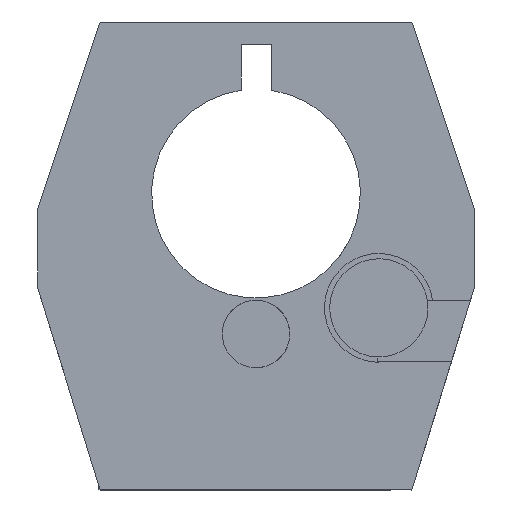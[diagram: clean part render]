
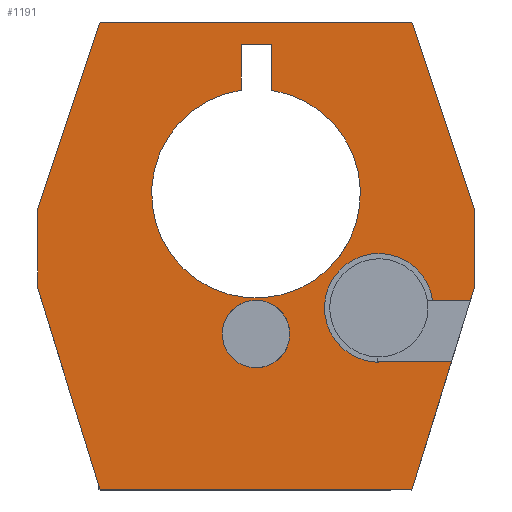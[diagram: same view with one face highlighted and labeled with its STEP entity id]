
A CAD part, front view. The second image highlights one B-rep face of the part: STEP entity #1191.
In plain terms, the highlighted planar face has unit normal (0, -1, 0).
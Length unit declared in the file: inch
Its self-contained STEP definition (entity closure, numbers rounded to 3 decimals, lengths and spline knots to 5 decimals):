
#20=FACE_BOUND('',#128,.T.);
#21=FACE_BOUND('',#129,.T.);
#63=FACE_OUTER_BOUND('',#127,.T.);
#127=EDGE_LOOP('',(#891,#892,#893,#894,#895,#896,#897,#898,#899,#900,#901,
#902,#903,#904,#905,#906));
#128=EDGE_LOOP('',(#907,#908,#909,#910));
#129=EDGE_LOOP('',(#911,#912));
#177=CIRCLE('',#1270,0.10827);
#178=CIRCLE('',#1271,0.10827);
#180=CIRCLE('',#1280,0.17421);
#181=CIRCLE('',#1282,0.33465);
#190=LINE('',#1648,#342);
#239=LINE('',#1763,#391);
#243=LINE('',#1770,#395);
#248=LINE('',#1830,#400);
#250=LINE('',#1836,#402);
#251=LINE('',#1838,#403);
#252=LINE('',#1840,#404);
#253=LINE('',#1842,#405);
#254=LINE('',#1844,#406);
#255=LINE('',#1846,#407);
#256=LINE('',#1848,#408);
#257=LINE('',#1850,#409);
#258=LINE('',#1851,#410);
#259=LINE('',#1853,#411);
#260=LINE('',#1854,#412);
#261=LINE('',#1859,#413);
#262=LINE('',#1861,#414);
#263=LINE('',#1862,#415);
#342=VECTOR('',#1333,0.3937);
#391=VECTOR('',#1432,0.3937);
#395=VECTOR('',#1438,0.3937);
#400=VECTOR('',#1463,0.3937);
#402=VECTOR('',#1471,0.3937);
#403=VECTOR('',#1472,0.3937);
#404=VECTOR('',#1473,0.3937);
#405=VECTOR('',#1474,0.3937);
#406=VECTOR('',#1475,0.3937);
#407=VECTOR('',#1476,0.3937);
#408=VECTOR('',#1477,0.3937);
#409=VECTOR('',#1478,0.3937);
#410=VECTOR('',#1479,0.3937);
#411=VECTOR('',#1480,0.3937);
#412=VECTOR('',#1481,0.3937);
#413=VECTOR('',#1484,0.3937);
#414=VECTOR('',#1485,0.3937);
#415=VECTOR('',#1486,0.3937);
#494=VERTEX_POINT('',#1645);
#495=VERTEX_POINT('',#1647);
#535=VERTEX_POINT('',#1760);
#536=VERTEX_POINT('',#1762);
#538=VERTEX_POINT('',#1768);
#539=VERTEX_POINT('',#1772);
#540=VERTEX_POINT('',#1773);
#546=VERTEX_POINT('',#1827);
#547=VERTEX_POINT('',#1829);
#548=VERTEX_POINT('',#1835);
#549=VERTEX_POINT('',#1837);
#550=VERTEX_POINT('',#1839);
#551=VERTEX_POINT('',#1841);
#552=VERTEX_POINT('',#1843);
#553=VERTEX_POINT('',#1845);
#554=VERTEX_POINT('',#1847);
#555=VERTEX_POINT('',#1849);
#556=VERTEX_POINT('',#1852);
#557=VERTEX_POINT('',#1855);
#558=VERTEX_POINT('',#1856);
#559=VERTEX_POINT('',#1858);
#560=VERTEX_POINT('',#1860);
#608=EDGE_CURVE('',#495,#494,#190,.T.);
#663=EDGE_CURVE('',#535,#536,#239,.T.);
#667=EDGE_CURVE('',#538,#535,#243,.T.);
#668=EDGE_CURVE('',#539,#540,#177,.T.);
#669=EDGE_CURVE('',#540,#539,#178,.T.);
#679=EDGE_CURVE('',#547,#546,#248,.T.);
#681=EDGE_CURVE('',#494,#547,#180,.T.);
#682=EDGE_CURVE('',#546,#548,#250,.T.);
#683=EDGE_CURVE('',#548,#549,#251,.T.);
#684=EDGE_CURVE('',#549,#550,#252,.T.);
#685=EDGE_CURVE('',#550,#551,#253,.T.);
#686=EDGE_CURVE('',#551,#552,#254,.T.);
#687=EDGE_CURVE('',#552,#553,#255,.T.);
#688=EDGE_CURVE('',#553,#554,#256,.T.);
#689=EDGE_CURVE('',#554,#555,#257,.T.);
#690=EDGE_CURVE('',#555,#536,#258,.T.);
#691=EDGE_CURVE('',#538,#556,#259,.T.);
#692=EDGE_CURVE('',#556,#495,#260,.T.);
#693=EDGE_CURVE('',#557,#558,#181,.T.);
#694=EDGE_CURVE('',#558,#559,#261,.T.);
#695=EDGE_CURVE('',#559,#560,#262,.T.);
#696=EDGE_CURVE('',#560,#557,#263,.T.);
#891=ORIENTED_EDGE('',*,*,#608,.T.);
#892=ORIENTED_EDGE('',*,*,#681,.T.);
#893=ORIENTED_EDGE('',*,*,#679,.T.);
#894=ORIENTED_EDGE('',*,*,#682,.T.);
#895=ORIENTED_EDGE('',*,*,#683,.T.);
#896=ORIENTED_EDGE('',*,*,#684,.T.);
#897=ORIENTED_EDGE('',*,*,#685,.T.);
#898=ORIENTED_EDGE('',*,*,#686,.T.);
#899=ORIENTED_EDGE('',*,*,#687,.T.);
#900=ORIENTED_EDGE('',*,*,#688,.T.);
#901=ORIENTED_EDGE('',*,*,#689,.T.);
#902=ORIENTED_EDGE('',*,*,#690,.T.);
#903=ORIENTED_EDGE('',*,*,#663,.F.);
#904=ORIENTED_EDGE('',*,*,#667,.F.);
#905=ORIENTED_EDGE('',*,*,#691,.T.);
#906=ORIENTED_EDGE('',*,*,#692,.T.);
#907=ORIENTED_EDGE('',*,*,#693,.T.);
#908=ORIENTED_EDGE('',*,*,#694,.T.);
#909=ORIENTED_EDGE('',*,*,#695,.T.);
#910=ORIENTED_EDGE('',*,*,#696,.T.);
#911=ORIENTED_EDGE('',*,*,#668,.T.);
#912=ORIENTED_EDGE('',*,*,#669,.T.);
#1129=PLANE('',#1281);
#1191=ADVANCED_FACE('',(#63,#20,#21),#1129,.T.);
#1270=AXIS2_PLACEMENT_3D('',#1774,#1441,#1442);
#1271=AXIS2_PLACEMENT_3D('',#1775,#1443,#1444);
#1280=AXIS2_PLACEMENT_3D('',#1833,#1467,#1468);
#1281=AXIS2_PLACEMENT_3D('',#1834,#1469,#1470);
#1282=AXIS2_PLACEMENT_3D('',#1857,#1482,#1483);
#1333=DIRECTION('',(-1.,0.,0.));
#1432=DIRECTION('',(-1.,0.,0.));
#1438=DIRECTION('',(0.,0.,1.));
#1441=DIRECTION('center_axis',(0.,1.,0.));
#1442=DIRECTION('ref_axis',(1.,0.,0.));
#1443=DIRECTION('center_axis',(0.,1.,0.));
#1444=DIRECTION('ref_axis',(1.,0.,0.));
#1463=DIRECTION('',(1.,0.,0.));
#1467=DIRECTION('center_axis',(0.,1.,0.));
#1468=DIRECTION('ref_axis',(1.,0.,0.));
#1469=DIRECTION('center_axis',(0.,-1.,0.));
#1470=DIRECTION('ref_axis',(0.,0.,-1.));
#1471=DIRECTION('',(0.294,0.,0.956));
#1472=DIRECTION('',(0.,0.,1.));
#1473=DIRECTION('',(-0.316,0.,0.949));
#1474=DIRECTION('',(-1.,0.,0.));
#1475=DIRECTION('',(-0.316,0.,-0.949));
#1476=DIRECTION('',(0.,0.,-1.));
#1477=DIRECTION('',(0.294,0.,-0.956));
#1478=DIRECTION('',(0.294,0.,-0.956));
#1479=DIRECTION('',(0.,0.,1.));
#1480=DIRECTION('',(1.,0.,0.));
#1481=DIRECTION('',(0.294,0.,0.956));
#1482=DIRECTION('center_axis',(0.,1.,0.));
#1483=DIRECTION('ref_axis',(-1.,0.,0.));
#1484=DIRECTION('',(0.,0.,1.));
#1485=DIRECTION('',(1.,0.,0.));
#1486=DIRECTION('',(0.,0.,-1.));
#1645=CARTESIAN_POINT('',(0.41433,2.56,-0.08921));
#1647=CARTESIAN_POINT('',(0.6264,2.56,-0.08921));
#1648=CARTESIAN_POINT('',(0.10264,2.56,-0.08921));
#1760=CARTESIAN_POINT('',(0.43,2.56,-0.49997));
#1762=CARTESIAN_POINT('',(-0.5,2.56,-0.49997));
#1763=CARTESIAN_POINT('',(-0.14192,2.56,-0.49997));
#1768=CARTESIAN_POINT('',(0.43,2.56,-0.5));
#1770=CARTESIAN_POINT('',(0.43,2.56,-0.5));
#1772=CARTESIAN_POINT('',(-0.05174,2.56,0.0951));
#1773=CARTESIAN_POINT('',(-0.10827,2.56,0.));
#1774=CARTESIAN_POINT('Origin',(0.,2.56,0.));
#1775=CARTESIAN_POINT('Origin',(0.,2.56,0.));
#1827=CARTESIAN_POINT('',(0.68699,2.56,0.10773));
#1829=CARTESIAN_POINT('',(0.56626,2.56,0.10773));
#1830=CARTESIAN_POINT('',(0.03313,2.56,0.10773));
#1833=CARTESIAN_POINT('Origin',(0.3937,2.56,0.08378));
#1834=CARTESIAN_POINT('Origin',(-0.5,2.56,0.29994));
#1835=CARTESIAN_POINT('',(0.7,2.56,0.15));
#1836=CARTESIAN_POINT('',(0.5,2.56,-0.5));
#1837=CARTESIAN_POINT('',(0.7,2.56,0.4));
#1838=CARTESIAN_POINT('',(0.7,2.56,0.15));
#1839=CARTESIAN_POINT('',(0.5,2.56,1.));
#1840=CARTESIAN_POINT('',(0.7,2.56,0.4));
#1841=CARTESIAN_POINT('',(-0.5,2.56,1.));
#1842=CARTESIAN_POINT('',(0.5,2.56,1.));
#1843=CARTESIAN_POINT('',(-0.7,2.56,0.4));
#1844=CARTESIAN_POINT('',(-0.7,2.56,0.4));
#1845=CARTESIAN_POINT('',(-0.7,2.56,0.15));
#1846=CARTESIAN_POINT('',(-0.7,2.56,0.4));
#1847=CARTESIAN_POINT('',(-0.60447,2.56,-0.16048));
#1848=CARTESIAN_POINT('',(-0.7,2.56,0.15));
#1849=CARTESIAN_POINT('',(-0.5,2.56,-0.5));
#1850=CARTESIAN_POINT('',(-0.60447,2.56,-0.16048));
#1851=CARTESIAN_POINT('',(-0.5,2.56,-0.5));
#1852=CARTESIAN_POINT('',(0.5,2.56,-0.5));
#1853=CARTESIAN_POINT('',(0.43,2.56,-0.5));
#1854=CARTESIAN_POINT('',(0.5,2.56,-0.5));
#1855=CARTESIAN_POINT('',(0.05072,2.56,0.78078));
#1856=CARTESIAN_POINT('',(-0.0477,2.56,0.78123));
#1857=CARTESIAN_POINT('Origin',(0.,2.56,0.45));
#1858=CARTESIAN_POINT('',(-0.0477,2.56,0.92834));
#1859=CARTESIAN_POINT('',(-0.0477,2.56,0.54213));
#1860=CARTESIAN_POINT('',(0.05072,2.56,0.92834));
#1861=CARTESIAN_POINT('',(-0.22464,2.56,0.92834));
#1862=CARTESIAN_POINT('',(0.05072,2.56,0.46835));
